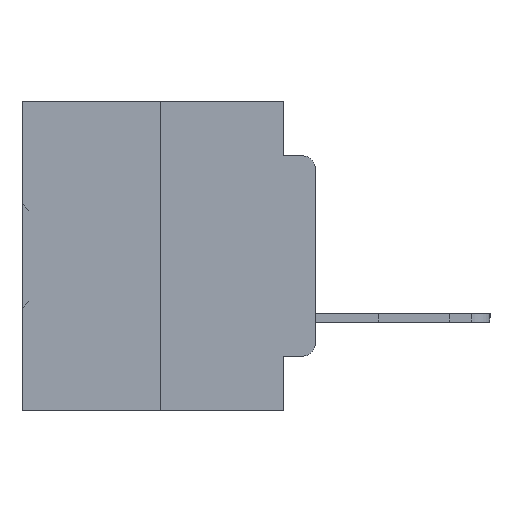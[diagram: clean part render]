
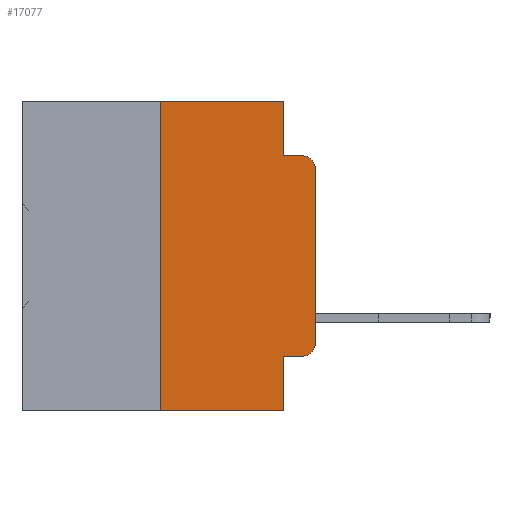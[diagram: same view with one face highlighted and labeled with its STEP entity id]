
A CAD part, left-side view. The second image highlights one B-rep face of the part: STEP entity #17077.
In plain terms, the highlighted planar face has unit normal (-1, 0, 0).
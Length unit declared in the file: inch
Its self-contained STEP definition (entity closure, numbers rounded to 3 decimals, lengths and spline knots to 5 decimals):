
#458 = VERTEX_POINT ( 'NONE', #35437 ) ;
#554 = VERTEX_POINT ( 'NONE', #1877 ) ;
#1282 = VERTEX_POINT ( 'NONE', #15014 ) ;
#1329 = CARTESIAN_POINT ( 'NONE',  ( 0., 0.25, 0. ) ) ;
#1877 = CARTESIAN_POINT ( 'NONE',  ( 0., 0., -0.3915 ) ) ;
#1969 = DIRECTION ( 'NONE',  ( 0., 0., 1. ) ) ;
#2007 = VERTEX_POINT ( 'NONE', #29291 ) ;
#2685 = CARTESIAN_POINT ( 'NONE',  ( 0., 0.02, -0.1085 ) ) ;
#2865 = DIRECTION ( 'NONE',  ( 0., -1., 0. ) ) ;
#2925 = CIRCLE ( 'NONE', #10685, 0.02 ) ;
#3029 = VECTOR ( 'NONE', #33067, 39.37008 ) ;
#3229 = VECTOR ( 'NONE', #37578, 39.37008 ) ;
#3738 = VERTEX_POINT ( 'NONE', #7728 ) ;
#3957 = DIRECTION ( 'NONE',  ( -1., 0., 0. ) ) ;
#4188 = AXIS2_PLACEMENT_3D ( 'NONE', #2685, #23077, #5612 ) ;
#4258 = DIRECTION ( 'NONE',  ( 0., 0., 1. ) ) ;
#4505 = ORIENTED_EDGE ( 'NONE', *, *, #16774, .T. ) ;
#4618 = CARTESIAN_POINT ( 'NONE',  ( 0., 0.473, -0.5 ) ) ;
#4646 = VECTOR ( 'NONE', #4258, 39.37008 ) ;
#4835 = EDGE_LOOP ( 'NONE', ( #8748, #4505, #24554, #5225, #20784, #24279, #21084, #26389, #32756, #13634 ) ) ;
#4900 = CARTESIAN_POINT ( 'NONE',  ( 0., 0., 0. ) ) ;
#5039 = EDGE_CURVE ( 'NONE', #458, #17323, #21178, .T. ) ;
#5225 = ORIENTED_EDGE ( 'NONE', *, *, #12897, .F. ) ;
#5612 = DIRECTION ( 'NONE',  ( 0., 0., -1. ) ) ;
#6647 = VECTOR ( 'NONE', #10493, 39.37008 ) ;
#7021 = EDGE_CURVE ( 'NONE', #458, #18780, #18716, .T. ) ;
#7510 = CARTESIAN_POINT ( 'NONE',  ( 0., 0.473, 0. ) ) ;
#7728 = CARTESIAN_POINT ( 'NONE',  ( 0., 0.051, -0.0885 ) ) ;
#8748 = ORIENTED_EDGE ( 'NONE', *, *, #24582, .T. ) ;
#8974 = EDGE_CURVE ( 'NONE', #26184, #22081, #27867, .T. ) ;
#10234 = DIRECTION ( 'NONE',  ( 0., -1., 0. ) ) ;
#10493 = DIRECTION ( 'NONE',  ( 0., -1., 0. ) ) ;
#10685 = AXIS2_PLACEMENT_3D ( 'NONE', #21437, #3957, #24351 ) ;
#10827 = CARTESIAN_POINT ( 'NONE',  ( 0., 0.051, 0. ) ) ;
#12524 = VECTOR ( 'NONE', #30215, 39.37008 ) ;
#12620 = VERTEX_POINT ( 'NONE', #10827 ) ;
#12897 = EDGE_CURVE ( 'NONE', #12620, #3738, #26226, .T. ) ;
#13634 = ORIENTED_EDGE ( 'NONE', *, *, #36927, .T. ) ;
#14844 = EDGE_CURVE ( 'NONE', #3738, #1282, #28985, .T. ) ;
#15014 = CARTESIAN_POINT ( 'NONE',  ( 0., 0.02, -0.0885 ) ) ;
#16191 = VECTOR ( 'NONE', #2865, 39.37008 ) ;
#16298 = PLANE ( 'NONE',  #19085 ) ;
#16329 = EDGE_CURVE ( 'NONE', #22081, #12620, #23037, .T. ) ;
#16774 = EDGE_CURVE ( 'NONE', #2007, #1282, #37451, .T. ) ;
#17077 = ADVANCED_FACE ( 'NONE', ( #35209 ), #16298, .F. ) ;
#17323 = VERTEX_POINT ( 'NONE', #26182 ) ;
#18716 = LINE ( 'NONE', #20140, #3229 ) ;
#18780 = VERTEX_POINT ( 'NONE', #35731 ) ;
#19085 = AXIS2_PLACEMENT_3D ( 'NONE', #7510, #36585, #19227 ) ;
#19227 = DIRECTION ( 'NONE',  ( 0., 0., -1. ) ) ;
#20140 = CARTESIAN_POINT ( 'NONE',  ( 0., 0.051, 0. ) ) ;
#20784 = ORIENTED_EDGE ( 'NONE', *, *, #16329, .F. ) ;
#21084 = ORIENTED_EDGE ( 'NONE', *, *, #25070, .T. ) ;
#21178 = LINE ( 'NONE', #32988, #12524 ) ;
#21276 = VECTOR ( 'NONE', #10234, 39.37008 ) ;
#21437 = CARTESIAN_POINT ( 'NONE',  ( 0., 0.02, -0.3915 ) ) ;
#22081 = VERTEX_POINT ( 'NONE', #36041 ) ;
#23037 = LINE ( 'NONE', #37636, #16191 ) ;
#23077 = DIRECTION ( 'NONE',  ( -1., 0., 0. ) ) ;
#24007 = VECTOR ( 'NONE', #1969, 39.37008 ) ;
#24279 = ORIENTED_EDGE ( 'NONE', *, *, #8974, .F. ) ;
#24351 = DIRECTION ( 'NONE',  ( 0., 0., -1. ) ) ;
#24554 = ORIENTED_EDGE ( 'NONE', *, *, #14844, .F. ) ;
#24582 = EDGE_CURVE ( 'NONE', #554, #2007, #31721, .T. ) ;
#25070 = EDGE_CURVE ( 'NONE', #26184, #18780, #29893, .T. ) ;
#26182 = CARTESIAN_POINT ( 'NONE',  ( 0., 0.02, -0.4115 ) ) ;
#26184 = VERTEX_POINT ( 'NONE', #33945 ) ;
#26226 = LINE ( 'NONE', #27224, #3029 ) ;
#26389 = ORIENTED_EDGE ( 'NONE', *, *, #7021, .F. ) ;
#27224 = CARTESIAN_POINT ( 'NONE',  ( 0., 0.051, 0. ) ) ;
#27645 = CARTESIAN_POINT ( 'NONE',  ( 0., 0.051, -0.0885 ) ) ;
#27867 = LINE ( 'NONE', #1329, #4646 ) ;
#28985 = LINE ( 'NONE', #27645, #21276 ) ;
#29291 = CARTESIAN_POINT ( 'NONE',  ( 0., 0., -0.1085 ) ) ;
#29893 = LINE ( 'NONE', #4618, #6647 ) ;
#30215 = DIRECTION ( 'NONE',  ( 0., -1., 0. ) ) ;
#31721 = LINE ( 'NONE', #4900, #24007 ) ;
#32756 = ORIENTED_EDGE ( 'NONE', *, *, #5039, .T. ) ;
#32988 = CARTESIAN_POINT ( 'NONE',  ( 0., 0.051, -0.4115 ) ) ;
#33067 = DIRECTION ( 'NONE',  ( 0., 0., -1. ) ) ;
#33945 = CARTESIAN_POINT ( 'NONE',  ( 0., 0.25, -0.5 ) ) ;
#35209 = FACE_OUTER_BOUND ( 'NONE', #4835, .T. ) ;
#35437 = CARTESIAN_POINT ( 'NONE',  ( 0., 0.051, -0.4115 ) ) ;
#35731 = CARTESIAN_POINT ( 'NONE',  ( 0., 0.051, -0.5 ) ) ;
#36041 = CARTESIAN_POINT ( 'NONE',  ( 0., 0.25, 0. ) ) ;
#36585 = DIRECTION ( 'NONE',  ( 1., 0., 0. ) ) ;
#36927 = EDGE_CURVE ( 'NONE', #17323, #554, #2925, .T. ) ;
#37451 = CIRCLE ( 'NONE', #4188, 0.02 ) ;
#37578 = DIRECTION ( 'NONE',  ( 0., 0., -1. ) ) ;
#37636 = CARTESIAN_POINT ( 'NONE',  ( 0., 0.473, 0. ) ) ;
